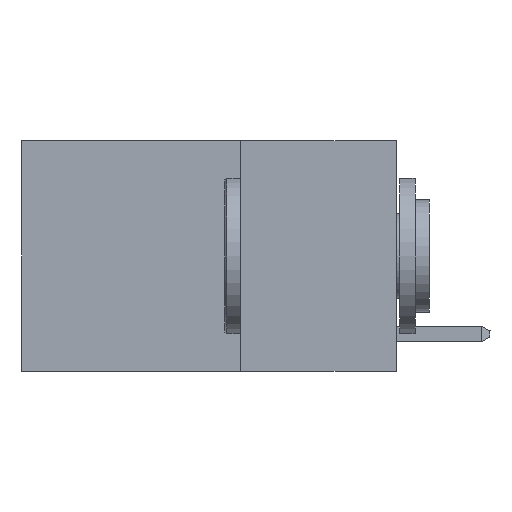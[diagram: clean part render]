
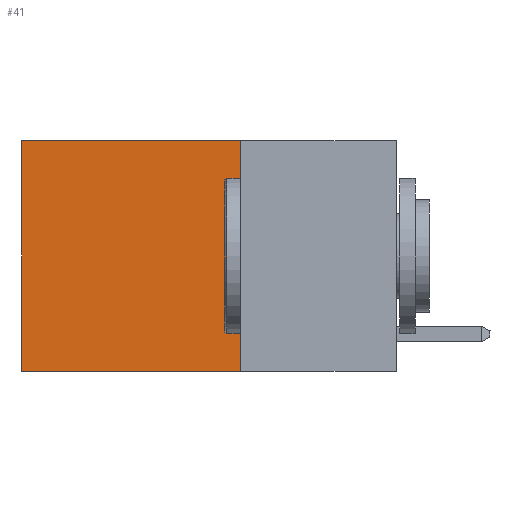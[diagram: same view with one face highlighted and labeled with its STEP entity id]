
A CAD part, left-side view. The second image highlights one B-rep face of the part: STEP entity #41.
In plain terms, the highlighted planar face has unit normal (-1, 0, 0).
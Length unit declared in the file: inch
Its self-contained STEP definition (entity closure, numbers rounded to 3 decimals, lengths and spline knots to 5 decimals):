
#41 = ADVANCED_FACE ( 'NONE', ( #11163 ), #652, .F. ) ;
#595 = LINE ( 'NONE', #23153, #12120 ) ;
#652 = PLANE ( 'NONE',  #23895 ) ;
#702 = CARTESIAN_POINT ( 'NONE',  ( 0.2625, 0.25, -0.37 ) ) ;
#2965 = CARTESIAN_POINT ( 'NONE',  ( 0.2625, 0.25, 0. ) ) ;
#5086 = EDGE_CURVE ( 'NONE', #29089, #6982, #21858, .T. ) ;
#5262 = DIRECTION ( 'NONE',  ( 1., 0., 0. ) ) ;
#6209 = CARTESIAN_POINT ( 'NONE',  ( 0.2625, 0.6, 0. ) ) ;
#6371 = EDGE_CURVE ( 'NONE', #23710, #16293, #16491, .T. ) ;
#6982 = VERTEX_POINT ( 'NONE', #10540 ) ;
#7393 = EDGE_CURVE ( 'NONE', #23710, #29089, #595, .T. ) ;
#7598 = DIRECTION ( 'NONE',  ( 0., 1., 0. ) ) ;
#8756 = CARTESIAN_POINT ( 'NONE',  ( 0.2625, 0.25, 0. ) ) ;
#10540 = CARTESIAN_POINT ( 'NONE',  ( 0.2625, 0.6, -0.37 ) ) ;
#10674 = CARTESIAN_POINT ( 'NONE',  ( 0.2625, 0.25, 0. ) ) ;
#11163 = FACE_OUTER_BOUND ( 'NONE', #14294, .T. ) ;
#11935 = DIRECTION ( 'NONE',  ( 0., 1., 0. ) ) ;
#12120 = VECTOR ( 'NONE', #11935, 39.37008 ) ;
#12531 = CARTESIAN_POINT ( 'NONE',  ( 0.2625, 0.25, -0.37 ) ) ;
#14294 = EDGE_LOOP ( 'NONE', ( #20254, #14925, #21657, #18213 ) ) ;
#14925 = ORIENTED_EDGE ( 'NONE', *, *, #26442, .F. ) ;
#16293 = VERTEX_POINT ( 'NONE', #12531 ) ;
#16491 = LINE ( 'NONE', #10674, #23189 ) ;
#18213 = ORIENTED_EDGE ( 'NONE', *, *, #7393, .T. ) ;
#20254 = ORIENTED_EDGE ( 'NONE', *, *, #5086, .T. ) ;
#21158 = VECTOR ( 'NONE', #24493, 39.37008 ) ;
#21283 = DIRECTION ( 'NONE',  ( 0., 0., -1. ) ) ;
#21657 = ORIENTED_EDGE ( 'NONE', *, *, #6371, .F. ) ;
#21858 = LINE ( 'NONE', #6209, #21158 ) ;
#22143 = VECTOR ( 'NONE', #7598, 39.37008 ) ;
#23153 = CARTESIAN_POINT ( 'NONE',  ( 0.2625, 0.25, 0. ) ) ;
#23189 = VECTOR ( 'NONE', #26606, 39.37008 ) ;
#23564 = LINE ( 'NONE', #702, #22143 ) ;
#23710 = VERTEX_POINT ( 'NONE', #8756 ) ;
#23895 = AXIS2_PLACEMENT_3D ( 'NONE', #2965, #5262, #21283 ) ;
#24493 = DIRECTION ( 'NONE',  ( 0., 0., -1. ) ) ;
#26442 = EDGE_CURVE ( 'NONE', #16293, #6982, #23564, .T. ) ;
#26606 = DIRECTION ( 'NONE',  ( 0., 0., -1. ) ) ;
#27927 = CARTESIAN_POINT ( 'NONE',  ( 0.2625, 0.6, 0. ) ) ;
#29089 = VERTEX_POINT ( 'NONE', #27927 ) ;
